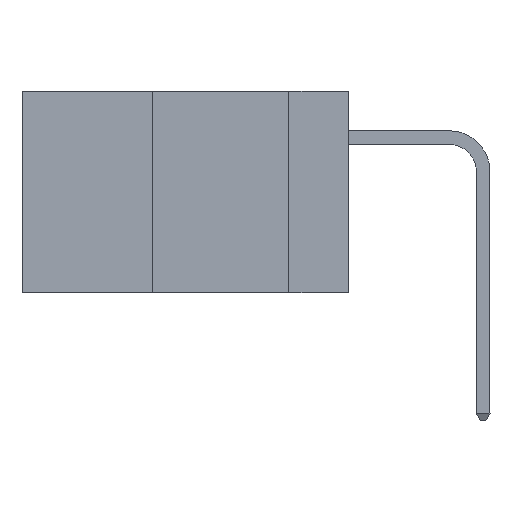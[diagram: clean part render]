
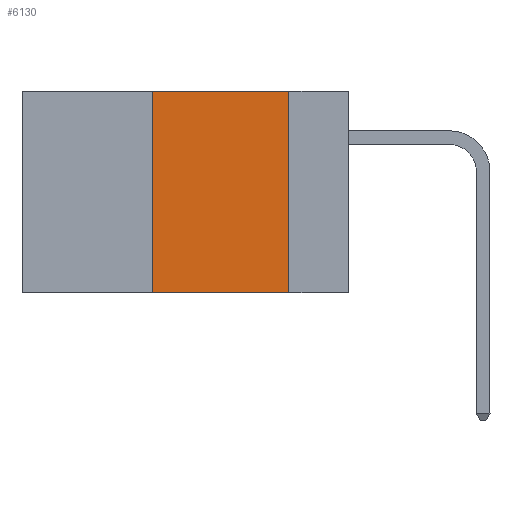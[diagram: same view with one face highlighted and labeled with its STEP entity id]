
A CAD part, left-side view. The second image highlights one B-rep face of the part: STEP entity #6130.
In plain terms, the highlighted planar face has unit normal (-1, 0, 0).
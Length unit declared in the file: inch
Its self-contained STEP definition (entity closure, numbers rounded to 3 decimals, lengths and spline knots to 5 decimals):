
#78 = VECTOR ( 'NONE', #8216, 39.37008 ) ;
#241 = ORIENTED_EDGE ( 'NONE', *, *, #8221, .F. ) ;
#600 = CARTESIAN_POINT ( 'NONE',  ( 0., 0.11, 0. ) ) ;
#1100 = VECTOR ( 'NONE', #10120, 39.37008 ) ;
#1340 = ORIENTED_EDGE ( 'NONE', *, *, #4412, .T. ) ;
#1415 = CARTESIAN_POINT ( 'NONE',  ( 0., 0.11, 0. ) ) ;
#2881 = EDGE_LOOP ( 'NONE', ( #3139, #241, #3217, #1340 ) ) ;
#2994 = VERTEX_POINT ( 'NONE', #8130 ) ;
#3139 = ORIENTED_EDGE ( 'NONE', *, *, #6194, .F. ) ;
#3217 = ORIENTED_EDGE ( 'NONE', *, *, #5206, .F. ) ;
#3327 = CARTESIAN_POINT ( 'NONE',  ( 0., 0.6, 0. ) ) ;
#3801 = DIRECTION ( 'NONE',  ( 0., 0., -1. ) ) ;
#4206 = LINE ( 'NONE', #3327, #9469 ) ;
#4221 = AXIS2_PLACEMENT_3D ( 'NONE', #10381, #6835, #3801 ) ;
#4243 = VECTOR ( 'NONE', #10102, 39.37008 ) ;
#4412 = EDGE_CURVE ( 'NONE', #2994, #11448, #11276, .T. ) ;
#4664 = PLANE ( 'NONE',  #4221 ) ;
#5206 = EDGE_CURVE ( 'NONE', #2994, #13685, #9919, .T. ) ;
#5504 = CARTESIAN_POINT ( 'NONE',  ( 0., 0.36, 0. ) ) ;
#6130 = ADVANCED_FACE ( 'NONE', ( #10240 ), #4664, .F. ) ;
#6194 = EDGE_CURVE ( 'NONE', #9348, #11448, #8149, .T. ) ;
#6588 = DIRECTION ( 'NONE',  ( 0., -1., 0. ) ) ;
#6835 = DIRECTION ( 'NONE',  ( 1., 0., 0. ) ) ;
#7213 = CARTESIAN_POINT ( 'NONE',  ( 0., 0.11, -0.37 ) ) ;
#8130 = CARTESIAN_POINT ( 'NONE',  ( 0., 0.36, -0.37 ) ) ;
#8149 = LINE ( 'NONE', #1415, #78 ) ;
#8216 = DIRECTION ( 'NONE',  ( 0., 0., -1. ) ) ;
#8221 = EDGE_CURVE ( 'NONE', #13685, #9348, #4206, .T. ) ;
#9320 = CARTESIAN_POINT ( 'NONE',  ( 0., 0.6, -0.37 ) ) ;
#9348 = VERTEX_POINT ( 'NONE', #600 ) ;
#9469 = VECTOR ( 'NONE', #6588, 39.37008 ) ;
#9919 = LINE ( 'NONE', #5504, #1100 ) ;
#10102 = DIRECTION ( 'NONE',  ( 0., -1., 0. ) ) ;
#10120 = DIRECTION ( 'NONE',  ( 0., 0., 1. ) ) ;
#10240 = FACE_OUTER_BOUND ( 'NONE', #2881, .T. ) ;
#10381 = CARTESIAN_POINT ( 'NONE',  ( 0., 0.6, 0. ) ) ;
#11276 = LINE ( 'NONE', #9320, #4243 ) ;
#11448 = VERTEX_POINT ( 'NONE', #7213 ) ;
#13532 = CARTESIAN_POINT ( 'NONE',  ( 0., 0.36, 0. ) ) ;
#13685 = VERTEX_POINT ( 'NONE', #13532 ) ;
